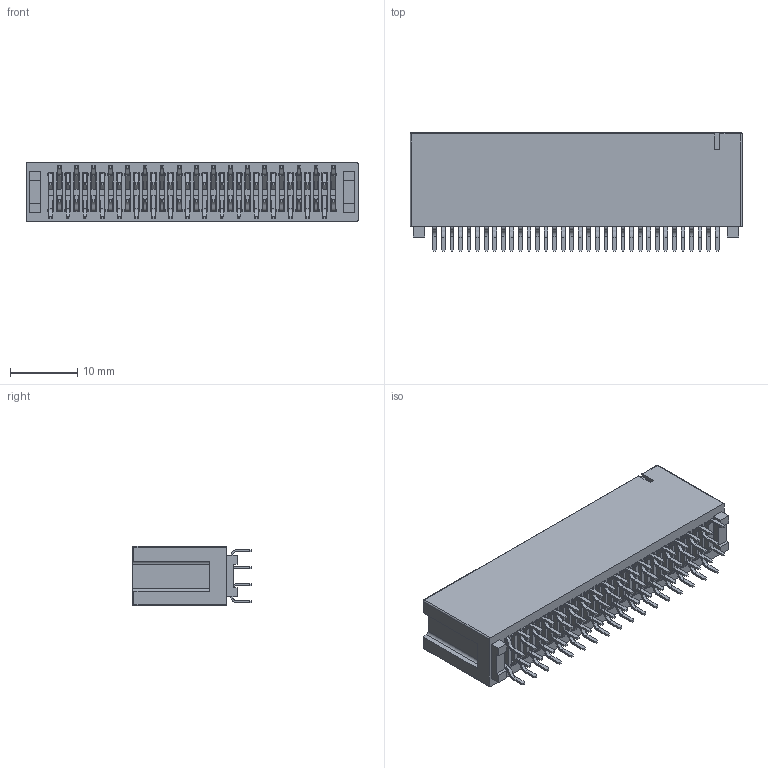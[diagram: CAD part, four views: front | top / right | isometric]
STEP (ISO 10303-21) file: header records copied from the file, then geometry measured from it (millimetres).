
FILE_DESCRIPTION (( 'STEP AP203' ), '1' );
FILE_NAME ('302-068-321-201.STEP', '2024-04-01T19:31:49', ( '' ), ( '' ), 'SwSTEP 2.0', 'SolidWorks 2023', '' );
FILE_SCHEMA (( 'CONFIG_CONTROL_DESIGN' ));
Length unit declared in the file: millimetre
Products named in the file (4): 302-068-321-201; HSG_Vertical HSG; Contact_302-290-X21 (1); Contact_302-290-X21 (2)
Assembly tree (69 placements, depth 2):
  302-068-321-201
    HSG_Vertical HSG
    Contact_302-290-X21 (2)  x34
    Contact_302-290-X21 (1)  x34
Bounding box: 49.28 x 17.63 x 8.88 mm (x, y, z)
Volume: 3836.3 mm3; surface area: 10459.6 mm2
Topology: 69 solids, 69 shells, 3160 faces, 9280 edges, 6088 vertices
Faces by surface type: plane 2327, cylinder 693, bspline 136, sphere 4
Entity records: 28196 total; most frequent: CARTESIAN_POINT 4840, ORIENTED_EDGE 4824, DIRECTION 3910, EDGE_CURVE 2412, LINE 2338, VECTOR 2338, VERTEX_POINT 1600, AXIS2_PLACEMENT_3D 786
